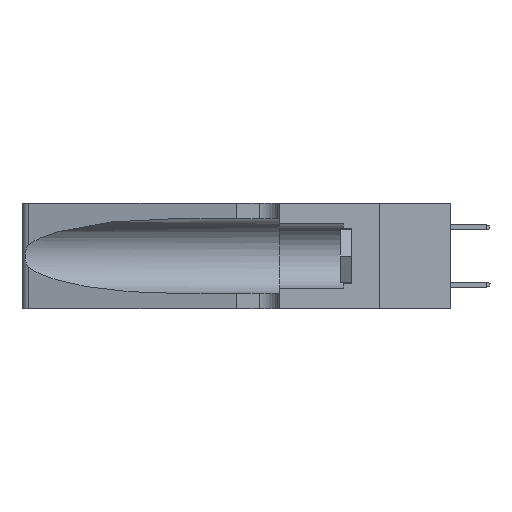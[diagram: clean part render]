
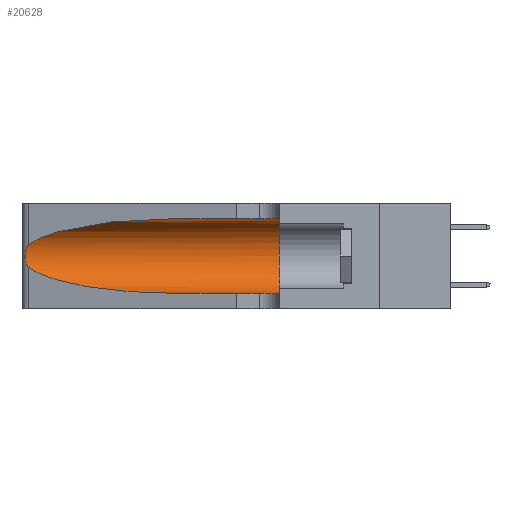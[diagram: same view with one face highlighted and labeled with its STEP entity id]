
A CAD part, left-side view. The second image highlights one B-rep face of the part: STEP entity #20628.
In plain terms, the highlighted cylindrical face has radius 3.308 mm (diameter 6.617 mm), a partial arc.
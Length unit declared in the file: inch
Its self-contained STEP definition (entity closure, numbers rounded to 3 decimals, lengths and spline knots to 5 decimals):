
#110 = CARTESIAN_POINT ( 'NONE',  ( 0.25487, 1.22718, 0.14631 ) ) ;
#415 = CARTESIAN_POINT ( 'NONE',  ( 0.26075, 1.23896, 0.19203 ) ) ;
#1002 = LINE ( 'NONE', #15215, #23108 ) ;
#1108 = CARTESIAN_POINT ( 'NONE',  ( 0.1305, 0.72297, 0.31525 ) ) ;
#1148 = CYLINDRICAL_SURFACE ( 'NONE', #14869, 0.13025 ) ;
#1779 = EDGE_CURVE ( 'NONE', #12780, #21348, #4586, .T. ) ;
#2007 = ORIENTED_EDGE ( 'NONE', *, *, #1779, .T. ) ;
#2133 = CARTESIAN_POINT ( 'NONE',  ( 0.1305, 0.35, 0.05475 ) ) ;
#2304 = VECTOR ( 'NONE', #11535, 39.37008 ) ;
#2330 = CARTESIAN_POINT ( 'NONE',  ( 0.25487, 1.22718, 0.22369 ) ) ;
#2795 = CARTESIAN_POINT ( 'NONE',  ( 0.2373, 1.15595, 0.08982 ) ) ;
#3644 = CARTESIAN_POINT ( 'NONE',  ( 0.25487, 1.22718, 0.22369 ) ) ;
#3690 = VERTEX_POINT ( 'NONE', #2133 ) ;
#4586 = B_SPLINE_CURVE_WITH_KNOTS ( 'NONE', 3,
 ( #2330, #16997, #5313, #29408, #26890, #21926, #415, #28780, #7063, #22076, #26560, #26725, #14948, #14294 ),
 .UNSPECIFIED., .F., .F.,
 ( 4, 2, 2, 2, 2, 2, 4 ),
 ( 0., 0.00027, 0.00053, 0.00107, 0.0016, 0.00187, 0.00214 ),
 .UNSPECIFIED. ) ;
#4696 = EDGE_CURVE ( 'NONE', #12868, #12780, #20589, .T. ) ;
#5313 = CARTESIAN_POINT ( 'NONE',  ( 0.25639, 1.23184, 0.21858 ) ) ;
#5995 = CARTESIAN_POINT ( 'NONE',  ( 0.2373, 1.15595, 0.28018 ) ) ;
#6355 = CARTESIAN_POINT ( 'NONE',  ( 0.1305, 1.61858, 0.05475 ) ) ;
#7063 = CARTESIAN_POINT ( 'NONE',  ( 0.26017, 1.23833, 0.17102 ) ) ;
#7110 = EDGE_LOOP ( 'NONE', ( #17358, #2007, #26617, #9636, #26766, #10904 ) ) ;
#7214 = CARTESIAN_POINT ( 'NONE',  ( 0.18966, 0.96281, 0.05475 ) ) ;
#8079 = EDGE_CURVE ( 'NONE', #20131, #3690, #19688, .T. ) ;
#8251 = FACE_OUTER_BOUND ( 'NONE', #7110, .T. ) ;
#8492 = DIRECTION ( 'NONE',  ( 0., 0., 1. ) ) ;
#9636 = ORIENTED_EDGE ( 'NONE', *, *, #21272, .T. ) ;
#9896 = CARTESIAN_POINT ( 'NONE',  ( 0.1305, 0.35, 0.31525 ) ) ;
#9897 = CARTESIAN_POINT ( 'NONE',  ( 0.1305, 0.72297, 0.05475 ) ) ;
#10286 = DIRECTION ( 'NONE',  ( 0., -1., 0. ) ) ;
#10629 = DIRECTION ( 'NONE',  ( 0., -1., 0. ) ) ;
#10754 = CARTESIAN_POINT ( 'NONE',  ( 0.1305, 1.61858, 0.185 ) ) ;
#10904 = ORIENTED_EDGE ( 'NONE', *, *, #29889, .F. ) ;
#11535 = DIRECTION ( 'NONE',  ( 0., -1., 0. ) ) ;
#12780 = VERTEX_POINT ( 'NONE', #30880 ) ;
#12862 = VERTEX_POINT ( 'NONE', #9897 ) ;
#12868 = VERTEX_POINT ( 'NONE', #24357 ) ;
#14294 = CARTESIAN_POINT ( 'NONE',  ( 0.25487, 1.22718, 0.14631 ) ) ;
#14627 = CARTESIAN_POINT ( 'NONE',  ( 0.1305, 0.72297, 0.05475 ) ) ;
#14869 = AXIS2_PLACEMENT_3D ( 'NONE', #10754, #10286, #30132 ) ;
#14948 = CARTESIAN_POINT ( 'NONE',  ( 0.25555, 1.22993, 0.14849 ) ) ;
#15215 = CARTESIAN_POINT ( 'NONE',  ( 0.1305, 1.61858, 0.31525 ) ) ;
#16997 = CARTESIAN_POINT ( 'NONE',  ( 0.25555, 1.22994, 0.2215 ) ) ;
#17358 = ORIENTED_EDGE ( 'NONE', *, *, #4696, .T. ) ;
#19688 = CIRCLE ( 'NONE', #23287, 0.13025 ) ;
#20131 = VERTEX_POINT ( 'NONE', #9896 ) ;
#20589 =( BOUNDED_CURVE ( )  B_SPLINE_CURVE ( 3, ( #1108, #27734, #5995, #3644 ),
 .UNSPECIFIED., .F., .T. ) 
 B_SPLINE_CURVE_WITH_KNOTS ( ( 4, 4 ),
 ( 1.5708, 2.84003 ),
 .UNSPECIFIED. ) 
 CURVE ( )  GEOMETRIC_REPRESENTATION_ITEM ( )  RATIONAL_B_SPLINE_CURVE ( ( 1., 0.87, 0.87, 1. ) ) 
 REPRESENTATION_ITEM ( '' )  );
#20628 = ADVANCED_FACE ( 'NONE', ( #8251 ), #1148, .F. ) ;
#21272 = EDGE_CURVE ( 'NONE', #12862, #3690, #28241, .T. ) ;
#21348 = VERTEX_POINT ( 'NONE', #27104 ) ;
#21926 = CARTESIAN_POINT ( 'NONE',  ( 0.26018, 1.23835, 0.19895 ) ) ;
#22076 = CARTESIAN_POINT ( 'NONE',  ( 0.25856, 1.23593, 0.16098 ) ) ;
#22303 = CARTESIAN_POINT ( 'NONE',  ( 0.1305, 0.35, 0.185 ) ) ;
#23108 = VECTOR ( 'NONE', #10629, 39.37008 ) ;
#23287 = AXIS2_PLACEMENT_3D ( 'NONE', #22303, #30227, #8492 ) ;
#23629 = EDGE_CURVE ( 'NONE', #21348, #12862, #25934, .T. ) ;
#24357 = CARTESIAN_POINT ( 'NONE',  ( 0.1305, 0.72297, 0.31525 ) ) ;
#25934 =( BOUNDED_CURVE ( )  B_SPLINE_CURVE ( 3, ( #110, #2795, #7214, #14627 ),
 .UNSPECIFIED., .F., .T. ) 
 B_SPLINE_CURVE_WITH_KNOTS ( ( 4, 4 ),
 ( 3.44316, 4.71239 ),
 .UNSPECIFIED. ) 
 CURVE ( )  GEOMETRIC_REPRESENTATION_ITEM ( )  RATIONAL_B_SPLINE_CURVE ( ( 1., 0.87, 0.87, 1. ) ) 
 REPRESENTATION_ITEM ( '' )  );
#26560 = CARTESIAN_POINT ( 'NONE',  ( 0.25789, 1.23486, 0.15765 ) ) ;
#26617 = ORIENTED_EDGE ( 'NONE', *, *, #23629, .T. ) ;
#26725 = CARTESIAN_POINT ( 'NONE',  ( 0.25639, 1.23186, 0.15144 ) ) ;
#26766 = ORIENTED_EDGE ( 'NONE', *, *, #8079, .F. ) ;
#26890 = CARTESIAN_POINT ( 'NONE',  ( 0.25854, 1.2359, 0.20912 ) ) ;
#27104 = CARTESIAN_POINT ( 'NONE',  ( 0.25487, 1.22718, 0.14631 ) ) ;
#27734 = CARTESIAN_POINT ( 'NONE',  ( 0.18966, 0.96281, 0.31525 ) ) ;
#28241 = LINE ( 'NONE', #6355, #2304 ) ;
#28780 = CARTESIAN_POINT ( 'NONE',  ( 0.26075, 1.23896, 0.178 ) ) ;
#29408 = CARTESIAN_POINT ( 'NONE',  ( 0.25787, 1.23484, 0.2124 ) ) ;
#29889 = EDGE_CURVE ( 'NONE', #12868, #20131, #1002, .T. ) ;
#30132 = DIRECTION ( 'NONE',  ( 0., 0., -1. ) ) ;
#30227 = DIRECTION ( 'NONE',  ( 0., 1., 0. ) ) ;
#30880 = CARTESIAN_POINT ( 'NONE',  ( 0.25487, 1.22718, 0.22369 ) ) ;
